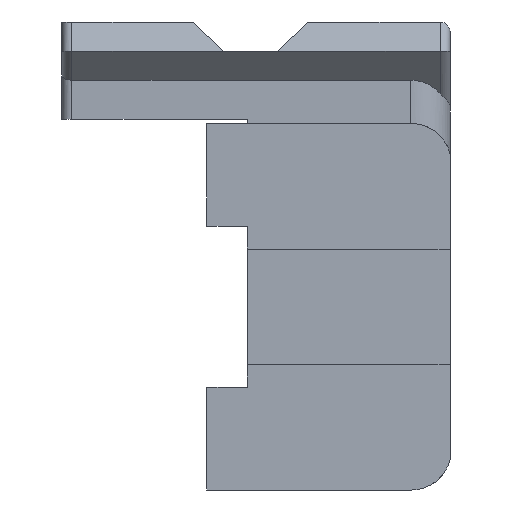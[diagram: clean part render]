
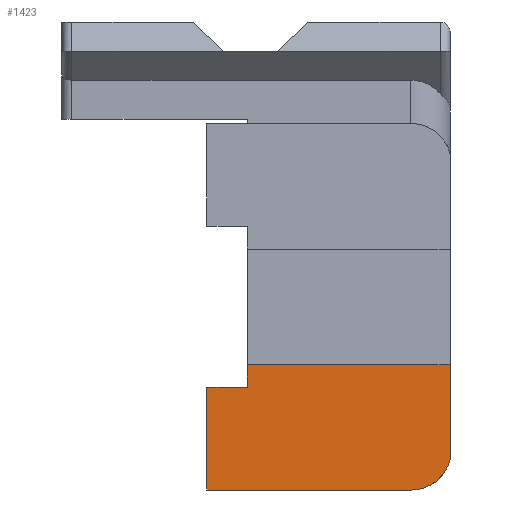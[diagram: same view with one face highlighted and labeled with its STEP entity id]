
A CAD part, front view. The second image highlights one B-rep face of the part: STEP entity #1423.
In plain terms, the highlighted planar face has unit normal (0, -1, 0).
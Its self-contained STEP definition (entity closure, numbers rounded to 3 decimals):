
#25 = EDGE_CURVE ( 'NONE', #2389, #1450, #1340, .T. ) ;
#153 = VECTOR ( 'NONE', #913, 1000. ) ;
#189 = VECTOR ( 'NONE', #1617, 1000. ) ;
#205 = CARTESIAN_POINT ( 'NONE',  ( 11.9, 100.06, -8.167 ) ) ;
#206 = VERTEX_POINT ( 'NONE', #2757 ) ;
#247 = AXIS2_PLACEMENT_3D ( 'NONE', #1427, #1891, #1908 ) ;
#301 = DIRECTION ( 'NONE',  ( 0., 0., -1. ) ) ;
#335 = EDGE_CURVE ( 'NONE', #1417, #1232, #784, .T. ) ;
#368 = AXIS2_PLACEMENT_3D ( 'NONE', #1369, #491, #1599 ) ;
#412 = ORIENTED_EDGE ( 'NONE', *, *, #1439, .T. ) ;
#438 = VECTOR ( 'NONE', #301, 1000. ) ;
#491 = DIRECTION ( 'NONE',  ( 0., -1., 0. ) ) ;
#496 = CARTESIAN_POINT ( 'NONE',  ( 9.5, 100.06, -8.167 ) ) ;
#527 = CARTESIAN_POINT ( 'NONE',  ( 32.528, 100.06, -18.549 ) ) ;
#640 = ORIENTED_EDGE ( 'NONE', *, *, #1056, .T. ) ;
#712 = CARTESIAN_POINT ( 'NONE',  ( 11.9, 100.06, -5.849 ) ) ;
#740 = CARTESIAN_POINT ( 'NONE',  ( 32.411, 100.06, -15.438 ) ) ;
#746 = LINE ( 'NONE', #1542, #153 ) ;
#784 = LINE ( 'NONE', #1230, #2444 ) ;
#876 = EDGE_CURVE ( 'NONE', #1351, #2389, #1899, .T. ) ;
#913 = DIRECTION ( 'NONE',  ( 0., 0., 1. ) ) ;
#935 = DIRECTION ( 'NONE',  ( -1., 0., 0. ) ) ;
#956 = LINE ( 'NONE', #1343, #2793 ) ;
#979 = ORIENTED_EDGE ( 'NONE', *, *, #25, .T. ) ;
#986 = DIRECTION ( 'NONE',  ( 1., 0., 0. ) ) ;
#1007 = CIRCLE ( 'NONE', #247, 4. ) ;
#1008 = CARTESIAN_POINT ( 'NONE',  ( 7.8, 100.06, -8.167 ) ) ;
#1056 = EDGE_CURVE ( 'NONE', #1417, #1351, #956, .T. ) ;
#1091 = FACE_OUTER_BOUND ( 'NONE', #1135, .T. ) ;
#1135 = EDGE_LOOP ( 'NONE', ( #412, #2373, #640, #2455, #979, #2775, #1397 ) ) ;
#1167 = CARTESIAN_POINT ( 'NONE',  ( 32.411, 100.06, -5.849 ) ) ;
#1230 = CARTESIAN_POINT ( 'NONE',  ( 5.35, 100.06, -5.849 ) ) ;
#1232 = VERTEX_POINT ( 'NONE', #1167 ) ;
#1237 = EDGE_CURVE ( 'NONE', #206, #1450, #2578, .T. ) ;
#1295 = VERTEX_POINT ( 'NONE', #740 ) ;
#1340 = LINE ( 'NONE', #1845, #438 ) ;
#1343 = CARTESIAN_POINT ( 'NONE',  ( 11.9, 100.06, 5.184 ) ) ;
#1351 = VERTEX_POINT ( 'NONE', #205 ) ;
#1369 = CARTESIAN_POINT ( 'NONE',  ( 11.7, 100.06, 18.535 ) ) ;
#1397 = ORIENTED_EDGE ( 'NONE', *, *, #2346, .F. ) ;
#1417 = VERTEX_POINT ( 'NONE', #712 ) ;
#1423 = ADVANCED_FACE ( 'NONE', ( #1091 ), #2741, .T. ) ;
#1427 = CARTESIAN_POINT ( 'NONE',  ( 28.511, 100.06, -14.549 ) ) ;
#1439 = EDGE_CURVE ( 'NONE', #1295, #1232, #746, .T. ) ;
#1450 = VERTEX_POINT ( 'NONE', #1583 ) ;
#1542 = CARTESIAN_POINT ( 'NONE',  ( 32.411, 100.06, 9.262 ) ) ;
#1583 = CARTESIAN_POINT ( 'NONE',  ( 7.8, 100.06, -18.549 ) ) ;
#1599 = DIRECTION ( 'NONE',  ( 1., 0., 0. ) ) ;
#1617 = DIRECTION ( 'NONE',  ( -1., 0., 0. ) ) ;
#1627 = VECTOR ( 'NONE', #935, 1000. ) ;
#1845 = CARTESIAN_POINT ( 'NONE',  ( 7.8, 100.06, 18.535 ) ) ;
#1891 = DIRECTION ( 'NONE',  ( 0., 1., 0. ) ) ;
#1899 = LINE ( 'NONE', #496, #1627 ) ;
#1908 = DIRECTION ( 'NONE',  ( 1., 0., 0. ) ) ;
#2346 = EDGE_CURVE ( 'NONE', #1295, #206, #1007, .T. ) ;
#2373 = ORIENTED_EDGE ( 'NONE', *, *, #335, .F. ) ;
#2389 = VERTEX_POINT ( 'NONE', #1008 ) ;
#2444 = VECTOR ( 'NONE', #986, 1000. ) ;
#2455 = ORIENTED_EDGE ( 'NONE', *, *, #876, .T. ) ;
#2578 = LINE ( 'NONE', #527, #189 ) ;
#2689 = DIRECTION ( 'NONE',  ( 0., 0., -1. ) ) ;
#2741 = PLANE ( 'NONE',  #368 ) ;
#2757 = CARTESIAN_POINT ( 'NONE',  ( 28.511, 100.06, -18.549 ) ) ;
#2775 = ORIENTED_EDGE ( 'NONE', *, *, #1237, .F. ) ;
#2793 = VECTOR ( 'NONE', #2689, 1000. ) ;
